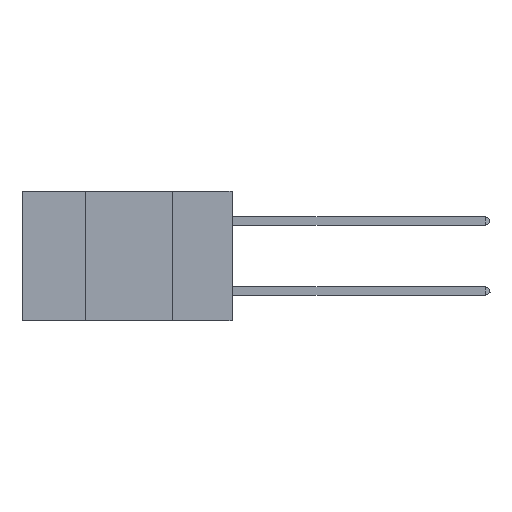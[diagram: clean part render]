
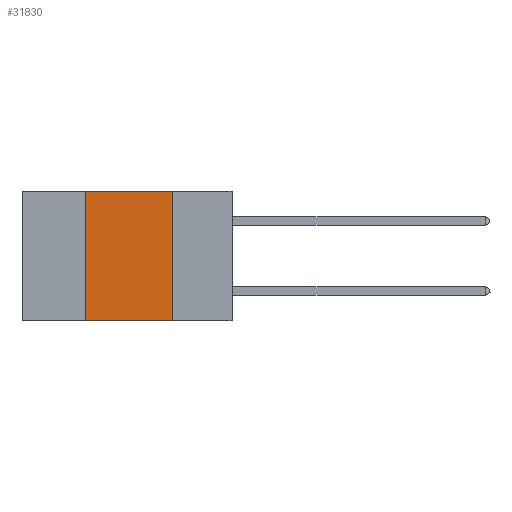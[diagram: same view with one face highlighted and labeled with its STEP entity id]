
A CAD part, left-side view. The second image highlights one B-rep face of the part: STEP entity #31830.
In plain terms, the highlighted planar face has unit normal (-1, 0, 0).
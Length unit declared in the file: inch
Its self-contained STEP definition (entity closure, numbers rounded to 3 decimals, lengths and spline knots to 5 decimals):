
#829 = CARTESIAN_POINT ( 'NONE',  ( 0., 0.6, 0. ) ) ;
#968 = PLANE ( 'NONE',  #26894 ) ;
#3871 = VECTOR ( 'NONE', #20829, 39.37008 ) ;
#4632 = EDGE_CURVE ( 'NONE', #20047, #32206, #22513, .T. ) ;
#9082 = CARTESIAN_POINT ( 'NONE',  ( 0., 0.17, -0.37 ) ) ;
#9324 = LINE ( 'NONE', #29704, #18250 ) ;
#9850 = ORIENTED_EDGE ( 'NONE', *, *, #43243, .F. ) ;
#10767 = EDGE_CURVE ( 'NONE', #20047, #28474, #37474, .T. ) ;
#13387 = CARTESIAN_POINT ( 'NONE',  ( 0., 0.42, 0. ) ) ;
#16257 = VERTEX_POINT ( 'NONE', #24546 ) ;
#18250 = VECTOR ( 'NONE', #39564, 39.37008 ) ;
#20047 = VERTEX_POINT ( 'NONE', #28914 ) ;
#20301 = FACE_OUTER_BOUND ( 'NONE', #31666, .T. ) ;
#20797 = DIRECTION ( 'NONE',  ( 0., -1., 0. ) ) ;
#20829 = DIRECTION ( 'NONE',  ( 0., 0., 1. ) ) ;
#22424 = ORIENTED_EDGE ( 'NONE', *, *, #10767, .F. ) ;
#22513 = LINE ( 'NONE', #42655, #25266 ) ;
#22783 = ORIENTED_EDGE ( 'NONE', *, *, #4632, .T. ) ;
#23159 = DIRECTION ( 'NONE',  ( 0., -1., 0. ) ) ;
#23938 = EDGE_CURVE ( 'NONE', #28474, #16257, #40305, .T. ) ;
#24173 = VECTOR ( 'NONE', #20797, 39.37008 ) ;
#24546 = CARTESIAN_POINT ( 'NONE',  ( 0., 0.17, 0. ) ) ;
#25266 = VECTOR ( 'NONE', #23159, 39.37008 ) ;
#26894 = AXIS2_PLACEMENT_3D ( 'NONE', #27298, #33443, #27517 ) ;
#27298 = CARTESIAN_POINT ( 'NONE',  ( 0., 0.6, 0. ) ) ;
#27517 = DIRECTION ( 'NONE',  ( 0., 0., -1. ) ) ;
#27849 = ORIENTED_EDGE ( 'NONE', *, *, #23938, .F. ) ;
#28474 = VERTEX_POINT ( 'NONE', #34251 ) ;
#28914 = CARTESIAN_POINT ( 'NONE',  ( 0., 0.42, -0.37 ) ) ;
#29704 = CARTESIAN_POINT ( 'NONE',  ( 0., 0.17, 0. ) ) ;
#31666 = EDGE_LOOP ( 'NONE', ( #9850, #27849, #22424, #22783 ) ) ;
#31830 = ADVANCED_FACE ( 'NONE', ( #20301 ), #968, .F. ) ;
#32206 = VERTEX_POINT ( 'NONE', #9082 ) ;
#33443 = DIRECTION ( 'NONE',  ( 1., 0., 0. ) ) ;
#34251 = CARTESIAN_POINT ( 'NONE',  ( 0., 0.42, 0. ) ) ;
#37474 = LINE ( 'NONE', #13387, #3871 ) ;
#39564 = DIRECTION ( 'NONE',  ( 0., 0., -1. ) ) ;
#40305 = LINE ( 'NONE', #829, #24173 ) ;
#42655 = CARTESIAN_POINT ( 'NONE',  ( 0., 0.6, -0.37 ) ) ;
#43243 = EDGE_CURVE ( 'NONE', #16257, #32206, #9324, .T. ) ;
